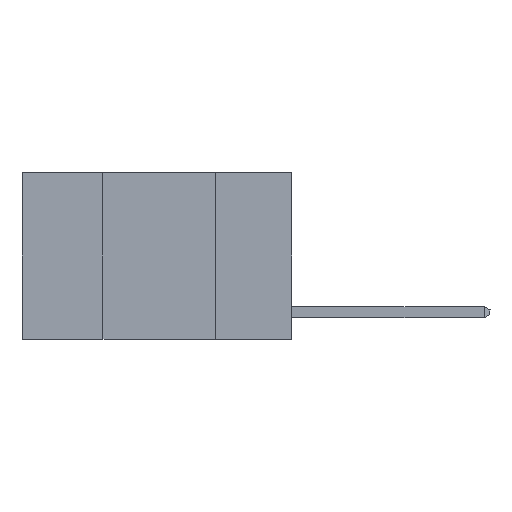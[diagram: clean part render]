
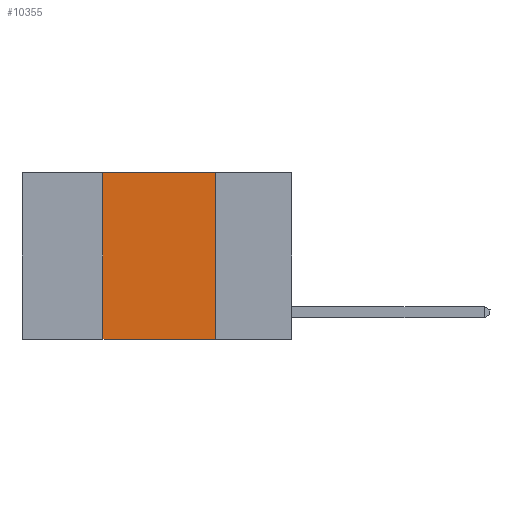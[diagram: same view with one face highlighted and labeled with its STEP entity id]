
A CAD part, left-side view. The second image highlights one B-rep face of the part: STEP entity #10355.
In plain terms, the highlighted planar face has unit normal (-1, 0, 0).
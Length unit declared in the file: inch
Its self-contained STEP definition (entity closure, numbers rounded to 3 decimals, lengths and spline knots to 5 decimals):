
#499 = VERTEX_POINT ( 'NONE', #2580 ) ;
#1193 = DIRECTION ( 'NONE',  ( 0., -1., 0. ) ) ;
#1215 = VECTOR ( 'NONE', #1513, 39.37008 ) ;
#1513 = DIRECTION ( 'NONE',  ( 0., 0., -1. ) ) ;
#1941 = DIRECTION ( 'NONE',  ( 0., -1., 0. ) ) ;
#2505 = ORIENTED_EDGE ( 'NONE', *, *, #3076, .F. ) ;
#2580 = CARTESIAN_POINT ( 'NONE',  ( 0., 0.17, 0. ) ) ;
#2856 = LINE ( 'NONE', #9504, #7808 ) ;
#3076 = EDGE_CURVE ( 'NONE', #7651, #9361, #6884, .T. ) ;
#4360 = CARTESIAN_POINT ( 'NONE',  ( 0., 0.17, 0. ) ) ;
#4420 = VECTOR ( 'NONE', #9467, 39.37008 ) ;
#4447 = ORIENTED_EDGE ( 'NONE', *, *, #6169, .F. ) ;
#4638 = CARTESIAN_POINT ( 'NONE',  ( 0., 0.42, 0. ) ) ;
#4657 = LINE ( 'NONE', #10141, #11449 ) ;
#5068 = ORIENTED_EDGE ( 'NONE', *, *, #8342, .T. ) ;
#5177 = DIRECTION ( 'NONE',  ( 0., 0., -1. ) ) ;
#5492 = VERTEX_POINT ( 'NONE', #6293 ) ;
#6169 = EDGE_CURVE ( 'NONE', #499, #5492, #8899, .T. ) ;
#6230 = FACE_OUTER_BOUND ( 'NONE', #6986, .T. ) ;
#6293 = CARTESIAN_POINT ( 'NONE',  ( 0., 0.17, -0.37 ) ) ;
#6884 = LINE ( 'NONE', #8555, #4420 ) ;
#6962 = PLANE ( 'NONE',  #7270 ) ;
#6986 = EDGE_LOOP ( 'NONE', ( #4447, #7198, #2505, #5068 ) ) ;
#7198 = ORIENTED_EDGE ( 'NONE', *, *, #8192, .F. ) ;
#7270 = AXIS2_PLACEMENT_3D ( 'NONE', #8743, #10480, #5177 ) ;
#7651 = VERTEX_POINT ( 'NONE', #8563 ) ;
#7808 = VECTOR ( 'NONE', #1193, 39.37008 ) ;
#8192 = EDGE_CURVE ( 'NONE', #9361, #499, #4657, .T. ) ;
#8342 = EDGE_CURVE ( 'NONE', #7651, #5492, #2856, .T. ) ;
#8555 = CARTESIAN_POINT ( 'NONE',  ( 0., 0.42, 0. ) ) ;
#8563 = CARTESIAN_POINT ( 'NONE',  ( 0., 0.42, -0.37 ) ) ;
#8743 = CARTESIAN_POINT ( 'NONE',  ( 0., 0.6, 0. ) ) ;
#8899 = LINE ( 'NONE', #4360, #1215 ) ;
#9361 = VERTEX_POINT ( 'NONE', #4638 ) ;
#9467 = DIRECTION ( 'NONE',  ( 0., 0., 1. ) ) ;
#9504 = CARTESIAN_POINT ( 'NONE',  ( 0., 0.6, -0.37 ) ) ;
#10141 = CARTESIAN_POINT ( 'NONE',  ( 0., 0.6, 0. ) ) ;
#10355 = ADVANCED_FACE ( 'NONE', ( #6230 ), #6962, .F. ) ;
#10480 = DIRECTION ( 'NONE',  ( 1., 0., 0. ) ) ;
#11449 = VECTOR ( 'NONE', #1941, 39.37008 ) ;
